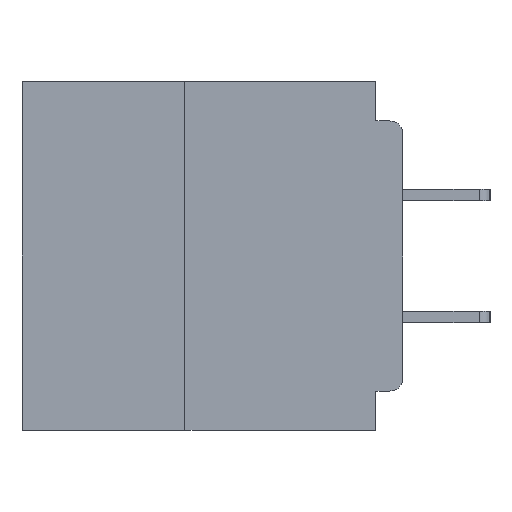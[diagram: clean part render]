
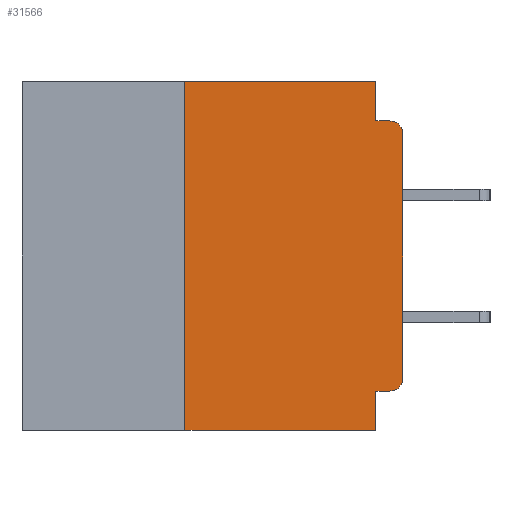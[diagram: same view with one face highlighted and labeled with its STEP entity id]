
A CAD part, left-side view. The second image highlights one B-rep face of the part: STEP entity #31566.
In plain terms, the highlighted planar face has unit normal (-1, 0, 0).
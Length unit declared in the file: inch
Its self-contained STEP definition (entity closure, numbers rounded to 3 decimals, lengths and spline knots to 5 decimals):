
#696 = CARTESIAN_POINT ( 'NONE',  ( 0., 0., -0.34 ) ) ;
#928 = EDGE_CURVE ( 'NONE', #25035, #5129, #7234, .T. ) ;
#1199 = CIRCLE ( 'NONE', #31823, 0.015 ) ;
#1438 = VERTEX_POINT ( 'NONE', #696 ) ;
#1458 = DIRECTION ( 'NONE',  ( 0., 0., -1. ) ) ;
#1619 = CARTESIAN_POINT ( 'NONE',  ( 0., 0.031, -0.4 ) ) ;
#1722 = ORIENTED_EDGE ( 'NONE', *, *, #27080, .T. ) ;
#3609 = LINE ( 'NONE', #30099, #18248 ) ;
#3836 = EDGE_CURVE ( 'NONE', #18322, #26891, #3609, .T. ) ;
#4837 = CARTESIAN_POINT ( 'NONE',  ( 0., 0.031, -0.4 ) ) ;
#4887 = LINE ( 'NONE', #17246, #33377 ) ;
#5129 = VERTEX_POINT ( 'NONE', #30117 ) ;
#6045 = CARTESIAN_POINT ( 'NONE',  ( 0., 0.031, 0. ) ) ;
#6099 = LINE ( 'NONE', #1619, #13414 ) ;
#6193 = ORIENTED_EDGE ( 'NONE', *, *, #8007, .T. ) ;
#6256 = DIRECTION ( 'NONE',  ( -1., 0., 0. ) ) ;
#6518 = ORIENTED_EDGE ( 'NONE', *, *, #26007, .F. ) ;
#6927 = CIRCLE ( 'NONE', #8955, 0.015 ) ;
#7234 = LINE ( 'NONE', #9642, #21025 ) ;
#7351 = ORIENTED_EDGE ( 'NONE', *, *, #10258, .F. ) ;
#7560 = DIRECTION ( 'NONE',  ( 0., 0., 1. ) ) ;
#8007 = EDGE_CURVE ( 'NONE', #28646, #14030, #1199, .T. ) ;
#8323 = DIRECTION ( 'NONE',  ( -1., 0., 0. ) ) ;
#8855 = EDGE_CURVE ( 'NONE', #1438, #28646, #31380, .T. ) ;
#8955 = AXIS2_PLACEMENT_3D ( 'NONE', #22762, #6256, #25532 ) ;
#8986 = CARTESIAN_POINT ( 'NONE',  ( 0., 0.437, 0. ) ) ;
#9374 = EDGE_LOOP ( 'NONE', ( #10914, #6193, #7351, #10857, #16364, #12526, #33522, #6518, #20502, #1722 ) ) ;
#9642 = CARTESIAN_POINT ( 'NONE',  ( 0., 0.031, 0. ) ) ;
#10088 = DIRECTION ( 'NONE',  ( 0., -1., 0. ) ) ;
#10202 = VECTOR ( 'NONE', #12472, 39.37008 ) ;
#10258 = EDGE_CURVE ( 'NONE', #5129, #14030, #11150, .T. ) ;
#10346 = VECTOR ( 'NONE', #7560, 39.37008 ) ;
#10745 = CARTESIAN_POINT ( 'NONE',  ( 0., 0., -0.06 ) ) ;
#10857 = ORIENTED_EDGE ( 'NONE', *, *, #928, .F. ) ;
#10914 = ORIENTED_EDGE ( 'NONE', *, *, #8855, .T. ) ;
#10977 = CARTESIAN_POINT ( 'NONE',  ( 0., 0.031, -0.355 ) ) ;
#11150 = LINE ( 'NONE', #32178, #24946 ) ;
#11786 = DIRECTION ( 'NONE',  ( 0., 0., -1. ) ) ;
#12472 = DIRECTION ( 'NONE',  ( 0., 0., 1. ) ) ;
#12526 = ORIENTED_EDGE ( 'NONE', *, *, #27416, .F. ) ;
#12595 = DIRECTION ( 'NONE',  ( 0., 0., -1. ) ) ;
#13181 = EDGE_CURVE ( 'NONE', #21182, #25035, #4887, .T. ) ;
#13414 = VECTOR ( 'NONE', #12595, 39.37008 ) ;
#13555 = DIRECTION ( 'NONE',  ( 0., 1., 0. ) ) ;
#14030 = VERTEX_POINT ( 'NONE', #22734 ) ;
#16357 = LINE ( 'NONE', #30669, #22833 ) ;
#16364 = ORIENTED_EDGE ( 'NONE', *, *, #13181, .F. ) ;
#17246 = CARTESIAN_POINT ( 'NONE',  ( 0., 0.437, 0. ) ) ;
#17858 = VERTEX_POINT ( 'NONE', #30400 ) ;
#18248 = VECTOR ( 'NONE', #13555, 39.37008 ) ;
#18322 = VERTEX_POINT ( 'NONE', #21526 ) ;
#19945 = PLANE ( 'NONE',  #20827 ) ;
#20502 = ORIENTED_EDGE ( 'NONE', *, *, #3836, .F. ) ;
#20827 = AXIS2_PLACEMENT_3D ( 'NONE', #8986, #28313, #11786 ) ;
#21025 = VECTOR ( 'NONE', #1458, 39.37008 ) ;
#21182 = VERTEX_POINT ( 'NONE', #29178 ) ;
#21526 = CARTESIAN_POINT ( 'NONE',  ( 0., 0.015, -0.355 ) ) ;
#22734 = CARTESIAN_POINT ( 'NONE',  ( 0., 0.015, -0.045 ) ) ;
#22762 = CARTESIAN_POINT ( 'NONE',  ( 0., 0.015, -0.34 ) ) ;
#22833 = VECTOR ( 'NONE', #25218, 39.37008 ) ;
#24785 = FACE_OUTER_BOUND ( 'NONE', #9374, .T. ) ;
#24819 = CARTESIAN_POINT ( 'NONE',  ( 0., 0.015, -0.06 ) ) ;
#24946 = VECTOR ( 'NONE', #10088, 39.37008 ) ;
#25022 = LINE ( 'NONE', #32406, #10346 ) ;
#25035 = VERTEX_POINT ( 'NONE', #6045 ) ;
#25218 = DIRECTION ( 'NONE',  ( 0., -1., 0. ) ) ;
#25532 = DIRECTION ( 'NONE',  ( 0., 0., -1. ) ) ;
#26007 = EDGE_CURVE ( 'NONE', #26891, #30467, #6099, .T. ) ;
#26891 = VERTEX_POINT ( 'NONE', #10977 ) ;
#27080 = EDGE_CURVE ( 'NONE', #18322, #1438, #6927, .T. ) ;
#27416 = EDGE_CURVE ( 'NONE', #17858, #21182, #25022, .T. ) ;
#27613 = DIRECTION ( 'NONE',  ( 0., 0., -1. ) ) ;
#28313 = DIRECTION ( 'NONE',  ( 1., 0., 0. ) ) ;
#28646 = VERTEX_POINT ( 'NONE', #10745 ) ;
#29026 = CARTESIAN_POINT ( 'NONE',  ( 0., 0., 0. ) ) ;
#29178 = CARTESIAN_POINT ( 'NONE',  ( 0., 0.25, 0. ) ) ;
#30099 = CARTESIAN_POINT ( 'NONE',  ( 0., 0., -0.355 ) ) ;
#30117 = CARTESIAN_POINT ( 'NONE',  ( 0., 0.031, -0.045 ) ) ;
#30400 = CARTESIAN_POINT ( 'NONE',  ( 0., 0.25, -0.4 ) ) ;
#30467 = VERTEX_POINT ( 'NONE', #4837 ) ;
#30669 = CARTESIAN_POINT ( 'NONE',  ( 0., 0.437, -0.4 ) ) ;
#31380 = LINE ( 'NONE', #29026, #10202 ) ;
#31566 = ADVANCED_FACE ( 'NONE', ( #24785 ), #19945, .F. ) ;
#31823 = AXIS2_PLACEMENT_3D ( 'NONE', #24819, #8323, #27613 ) ;
#32178 = CARTESIAN_POINT ( 'NONE',  ( 0., 0., -0.045 ) ) ;
#32406 = CARTESIAN_POINT ( 'NONE',  ( 0., 0.25, -0.4 ) ) ;
#33377 = VECTOR ( 'NONE', #33909, 39.37008 ) ;
#33522 = ORIENTED_EDGE ( 'NONE', *, *, #35323, .T. ) ;
#33909 = DIRECTION ( 'NONE',  ( 0., -1., 0. ) ) ;
#35323 = EDGE_CURVE ( 'NONE', #17858, #30467, #16357, .T. ) ;
